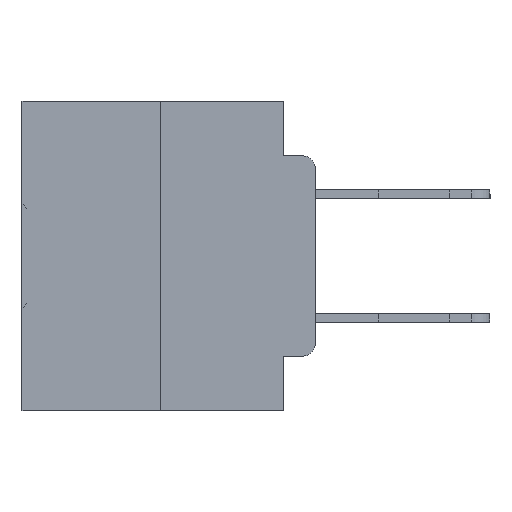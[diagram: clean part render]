
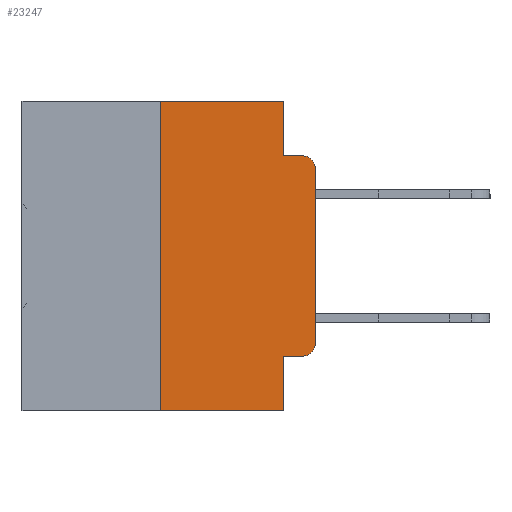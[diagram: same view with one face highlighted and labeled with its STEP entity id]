
A CAD part, left-side view. The second image highlights one B-rep face of the part: STEP entity #23247.
In plain terms, the highlighted planar face has unit normal (-1, 0, 0).
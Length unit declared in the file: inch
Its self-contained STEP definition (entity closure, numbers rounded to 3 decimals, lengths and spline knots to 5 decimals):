
#238 = ORIENTED_EDGE ( 'NONE', *, *, #30686, .F. ) ;
#386 = CARTESIAN_POINT ( 'NONE',  ( 0., 0.051, -0.4115 ) ) ;
#563 = VECTOR ( 'NONE', #14783, 39.37008 ) ;
#1101 = VECTOR ( 'NONE', #14843, 39.37008 ) ;
#1213 = DIRECTION ( 'NONE',  ( -1., 0., 0. ) ) ;
#1370 = VERTEX_POINT ( 'NONE', #18458 ) ;
#1596 = LINE ( 'NONE', #15592, #28625 ) ;
#2645 = ORIENTED_EDGE ( 'NONE', *, *, #25497, .T. ) ;
#2671 = EDGE_CURVE ( 'NONE', #29942, #15605, #22378, .T. ) ;
#4168 = CARTESIAN_POINT ( 'NONE',  ( 0., 0.25, 0. ) ) ;
#6279 = AXIS2_PLACEMENT_3D ( 'NONE', #26234, #13338, #31429 ) ;
#6499 = CARTESIAN_POINT ( 'NONE',  ( 0., 0.02, -0.4115 ) ) ;
#6594 = VERTEX_POINT ( 'NONE', #15029 ) ;
#6661 = EDGE_CURVE ( 'NONE', #29149, #12400, #29084, .T. ) ;
#7149 = CARTESIAN_POINT ( 'NONE',  ( 0., 0.051, -0.0885 ) ) ;
#7304 = EDGE_CURVE ( 'NONE', #9908, #1370, #1596, .T. ) ;
#7911 = EDGE_CURVE ( 'NONE', #11287, #12400, #10716, .T. ) ;
#8125 = VERTEX_POINT ( 'NONE', #6499 ) ;
#8144 = LINE ( 'NONE', #4168, #1101 ) ;
#8298 = VECTOR ( 'NONE', #16066, 39.37008 ) ;
#8457 = VECTOR ( 'NONE', #24629, 39.37008 ) ;
#9461 = CARTESIAN_POINT ( 'NONE',  ( 0., 0., -0.3915 ) ) ;
#9605 = CARTESIAN_POINT ( 'NONE',  ( 0., 0.473, 0. ) ) ;
#9908 = VERTEX_POINT ( 'NONE', #11301 ) ;
#10189 = ORIENTED_EDGE ( 'NONE', *, *, #24216, .T. ) ;
#10716 = LINE ( 'NONE', #25840, #23755 ) ;
#10916 = VECTOR ( 'NONE', #12540, 39.37008 ) ;
#11248 = ORIENTED_EDGE ( 'NONE', *, *, #6661, .F. ) ;
#11287 = VERTEX_POINT ( 'NONE', #11882 ) ;
#11301 = CARTESIAN_POINT ( 'NONE',  ( 0., 0.051, 0. ) ) ;
#11882 = CARTESIAN_POINT ( 'NONE',  ( 0., 0.25, -0.5 ) ) ;
#12400 = VERTEX_POINT ( 'NONE', #19325 ) ;
#12540 = DIRECTION ( 'NONE',  ( 0., -1., 0. ) ) ;
#12583 = EDGE_CURVE ( 'NONE', #6594, #9908, #28413, .T. ) ;
#13338 = DIRECTION ( 'NONE',  ( 1., 0., 0. ) ) ;
#13444 = ORIENTED_EDGE ( 'NONE', *, *, #28308, .F. ) ;
#13739 = DIRECTION ( 'NONE',  ( 0., -1., 0. ) ) ;
#13799 = ORIENTED_EDGE ( 'NONE', *, *, #7304, .F. ) ;
#14101 = AXIS2_PLACEMENT_3D ( 'NONE', #17048, #1213, #19660 ) ;
#14320 = DIRECTION ( 'NONE',  ( 0., 0., -1. ) ) ;
#14741 = CARTESIAN_POINT ( 'NONE',  ( 0., 0.02, -0.3915 ) ) ;
#14783 = DIRECTION ( 'NONE',  ( 0., -1., 0. ) ) ;
#14843 = DIRECTION ( 'NONE',  ( 0., 0., 1. ) ) ;
#15029 = CARTESIAN_POINT ( 'NONE',  ( 0., 0.25, 0. ) ) ;
#15592 = CARTESIAN_POINT ( 'NONE',  ( 0., 0.051, 0. ) ) ;
#15605 = VERTEX_POINT ( 'NONE', #26935 ) ;
#16066 = DIRECTION ( 'NONE',  ( 0., 0., -1. ) ) ;
#16171 = CIRCLE ( 'NONE', #20163, 0.02 ) ;
#16594 = ORIENTED_EDGE ( 'NONE', *, *, #2671, .T. ) ;
#16871 = ORIENTED_EDGE ( 'NONE', *, *, #12583, .F. ) ;
#17048 = CARTESIAN_POINT ( 'NONE',  ( 0., 0.02, -0.1085 ) ) ;
#17349 = DIRECTION ( 'NONE',  ( 0., 0., -1. ) ) ;
#17864 = LINE ( 'NONE', #7149, #10916 ) ;
#18024 = CARTESIAN_POINT ( 'NONE',  ( 0., 0.051, 0. ) ) ;
#18088 = VECTOR ( 'NONE', #13739, 39.37008 ) ;
#18166 = CIRCLE ( 'NONE', #14101, 0.02 ) ;
#18458 = CARTESIAN_POINT ( 'NONE',  ( 0., 0.051, -0.0885 ) ) ;
#18549 = ORIENTED_EDGE ( 'NONE', *, *, #19012, .T. ) ;
#19012 = EDGE_CURVE ( 'NONE', #29149, #8125, #24969, .T. ) ;
#19325 = CARTESIAN_POINT ( 'NONE',  ( 0., 0.051, -0.5 ) ) ;
#19484 = FACE_OUTER_BOUND ( 'NONE', #19571, .T. ) ;
#19571 = EDGE_LOOP ( 'NONE', ( #16594, #2645, #238, #13799, #16871, #13444, #31646, #11248, #18549, #10189 ) ) ;
#19660 = DIRECTION ( 'NONE',  ( 0., 0., -1. ) ) ;
#20163 = AXIS2_PLACEMENT_3D ( 'NONE', #14741, #32814, #17349 ) ;
#21065 = PLANE ( 'NONE',  #6279 ) ;
#21615 = CARTESIAN_POINT ( 'NONE',  ( 0., 0.051, -0.4115 ) ) ;
#21827 = VERTEX_POINT ( 'NONE', #33220 ) ;
#22378 = LINE ( 'NONE', #28347, #8457 ) ;
#23247 = ADVANCED_FACE ( 'NONE', ( #19484 ), #21065, .F. ) ;
#23755 = VECTOR ( 'NONE', #24178, 39.37008 ) ;
#24178 = DIRECTION ( 'NONE',  ( 0., -1., 0. ) ) ;
#24216 = EDGE_CURVE ( 'NONE', #8125, #29942, #16171, .T. ) ;
#24629 = DIRECTION ( 'NONE',  ( 0., 0., 1. ) ) ;
#24969 = LINE ( 'NONE', #386, #18088 ) ;
#25497 = EDGE_CURVE ( 'NONE', #15605, #21827, #18166, .T. ) ;
#25840 = CARTESIAN_POINT ( 'NONE',  ( 0., 0.473, -0.5 ) ) ;
#26234 = CARTESIAN_POINT ( 'NONE',  ( 0., 0.473, 0. ) ) ;
#26935 = CARTESIAN_POINT ( 'NONE',  ( 0., 0., -0.1085 ) ) ;
#28308 = EDGE_CURVE ( 'NONE', #11287, #6594, #8144, .T. ) ;
#28347 = CARTESIAN_POINT ( 'NONE',  ( 0., 0., 0. ) ) ;
#28413 = LINE ( 'NONE', #9605, #563 ) ;
#28625 = VECTOR ( 'NONE', #14320, 39.37008 ) ;
#29084 = LINE ( 'NONE', #18024, #8298 ) ;
#29149 = VERTEX_POINT ( 'NONE', #21615 ) ;
#29942 = VERTEX_POINT ( 'NONE', #9461 ) ;
#30686 = EDGE_CURVE ( 'NONE', #1370, #21827, #17864, .T. ) ;
#31429 = DIRECTION ( 'NONE',  ( 0., 0., -1. ) ) ;
#31646 = ORIENTED_EDGE ( 'NONE', *, *, #7911, .T. ) ;
#32814 = DIRECTION ( 'NONE',  ( -1., 0., 0. ) ) ;
#33220 = CARTESIAN_POINT ( 'NONE',  ( 0., 0.02, -0.0885 ) ) ;
